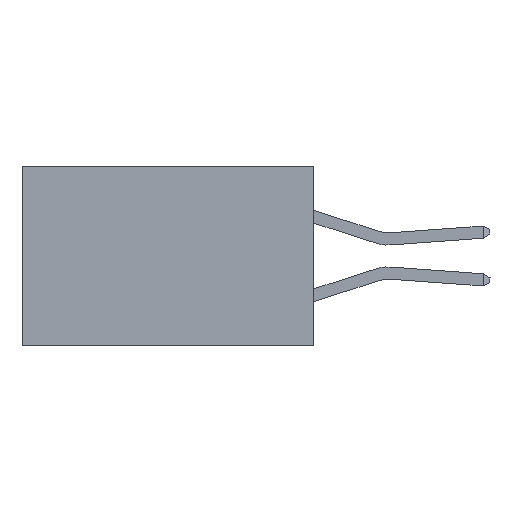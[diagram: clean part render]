
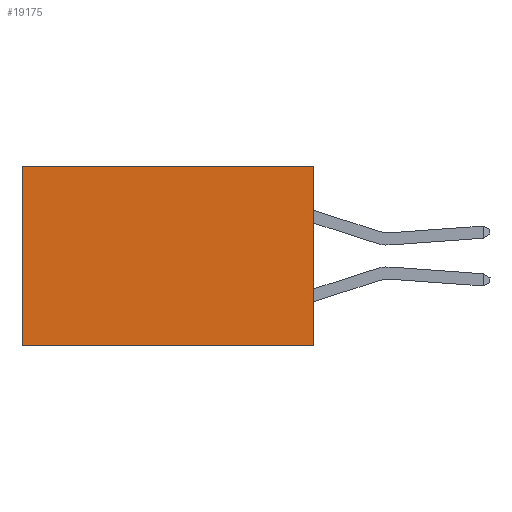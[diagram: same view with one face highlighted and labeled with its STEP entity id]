
A CAD part, left-side view. The second image highlights one B-rep face of the part: STEP entity #19175.
In plain terms, the highlighted planar face has unit normal (-1, 0, 0).
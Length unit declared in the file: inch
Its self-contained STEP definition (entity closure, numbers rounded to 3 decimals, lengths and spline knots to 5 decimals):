
#606 = DIRECTION ( 'NONE',  ( 0., 0., -1. ) ) ;
#620 = DIRECTION ( 'NONE',  ( 0., 1., 0. ) ) ;
#978 = DIRECTION ( 'NONE',  ( 0., 0., -1. ) ) ;
#1893 = CARTESIAN_POINT ( 'NONE',  ( 0.2875, 0., 0. ) ) ;
#2061 = DIRECTION ( 'NONE',  ( 1., 0., 0. ) ) ;
#2581 = ORIENTED_EDGE ( 'NONE', *, *, #15974, .T. ) ;
#4677 = ORIENTED_EDGE ( 'NONE', *, *, #7703, .T. ) ;
#4735 = LINE ( 'NONE', #22929, #15855 ) ;
#5206 = EDGE_LOOP ( 'NONE', ( #4677, #7269, #7558, #2581 ) ) ;
#6989 = CARTESIAN_POINT ( 'NONE',  ( 0.2875, 0.6, 0. ) ) ;
#7269 = ORIENTED_EDGE ( 'NONE', *, *, #13806, .F. ) ;
#7281 = VERTEX_POINT ( 'NONE', #12702 ) ;
#7492 = VERTEX_POINT ( 'NONE', #6989 ) ;
#7558 = ORIENTED_EDGE ( 'NONE', *, *, #17568, .F. ) ;
#7703 = EDGE_CURVE ( 'NONE', #7492, #7281, #12640, .T. ) ;
#7925 = FACE_OUTER_BOUND ( 'NONE', #5206, .T. ) ;
#8100 = VECTOR ( 'NONE', #24128, 39.37008 ) ;
#11231 = VECTOR ( 'NONE', #606, 39.37008 ) ;
#12640 = LINE ( 'NONE', #23566, #12966 ) ;
#12702 = CARTESIAN_POINT ( 'NONE',  ( 0.2875, 0.6, -0.37 ) ) ;
#12764 = AXIS2_PLACEMENT_3D ( 'NONE', #1893, #2061, #16272 ) ;
#12966 = VECTOR ( 'NONE', #978, 39.37008 ) ;
#13452 = LINE ( 'NONE', #16888, #11231 ) ;
#13806 = EDGE_CURVE ( 'NONE', #20364, #7281, #4735, .T. ) ;
#14201 = PLANE ( 'NONE',  #12764 ) ;
#14907 = VERTEX_POINT ( 'NONE', #20137 ) ;
#15855 = VECTOR ( 'NONE', #620, 39.37008 ) ;
#15974 = EDGE_CURVE ( 'NONE', #14907, #7492, #26228, .T. ) ;
#16272 = DIRECTION ( 'NONE',  ( 0., 0., -1. ) ) ;
#16888 = CARTESIAN_POINT ( 'NONE',  ( 0.2875, 0., 0. ) ) ;
#17568 = EDGE_CURVE ( 'NONE', #14907, #20364, #13452, .T. ) ;
#19175 = ADVANCED_FACE ( 'NONE', ( #7925 ), #14201, .F. ) ;
#20042 = CARTESIAN_POINT ( 'NONE',  ( 0.2875, 0., 0. ) ) ;
#20137 = CARTESIAN_POINT ( 'NONE',  ( 0.2875, 0., 0. ) ) ;
#20364 = VERTEX_POINT ( 'NONE', #22378 ) ;
#22378 = CARTESIAN_POINT ( 'NONE',  ( 0.2875, 0., -0.37 ) ) ;
#22929 = CARTESIAN_POINT ( 'NONE',  ( 0.2875, 0., -0.37 ) ) ;
#23566 = CARTESIAN_POINT ( 'NONE',  ( 0.2875, 0.6, 0. ) ) ;
#24128 = DIRECTION ( 'NONE',  ( 0., 1., 0. ) ) ;
#26228 = LINE ( 'NONE', #20042, #8100 ) ;
